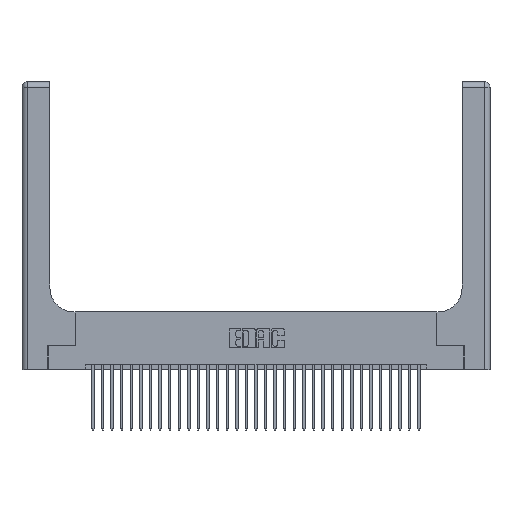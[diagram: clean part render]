
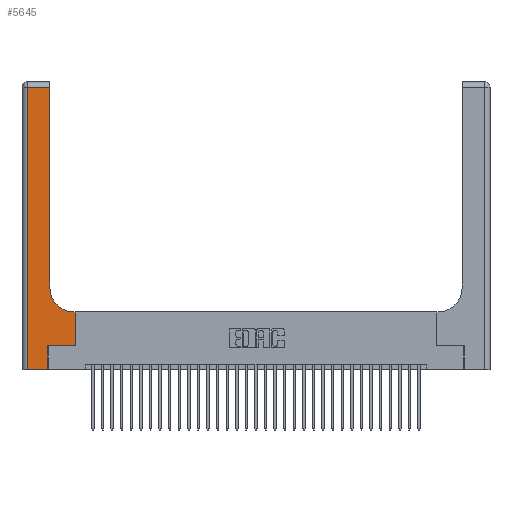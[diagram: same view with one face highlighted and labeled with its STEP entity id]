
A CAD part, top view. The second image highlights one B-rep face of the part: STEP entity #5645.
In plain terms, the highlighted planar face has unit normal (0, 0, 1).
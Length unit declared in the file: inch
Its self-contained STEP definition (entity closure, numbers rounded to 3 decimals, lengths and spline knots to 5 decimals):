
#362 = LINE ( 'NONE', #21223, #12542 ) ;
#438 = DIRECTION ( 'NONE',  ( -1., 0., 0. ) ) ;
#966 = LINE ( 'NONE', #25272, #27341 ) ;
#1006 = VECTOR ( 'NONE', #29697, 39.37008 ) ;
#2034 = CARTESIAN_POINT ( 'NONE',  ( 0., 3., 0.37 ) ) ;
#2257 = DIRECTION ( 'NONE',  ( 0., 0., -1. ) ) ;
#2410 = LINE ( 'NONE', #11811, #5665 ) ;
#4668 = LINE ( 'NONE', #6805, #24555 ) ;
#4976 = PLANE ( 'NONE',  #11623 ) ;
#5116 = AXIS2_PLACEMENT_3D ( 'NONE', #25966, #2257, #20649 ) ;
#5642 = CARTESIAN_POINT ( 'NONE',  ( 0.5585, 0.6, 0.37 ) ) ;
#5645 = ADVANCED_FACE ( 'NONE', ( #11794 ), #4976, .F. ) ;
#5660 = DIRECTION ( 'NONE',  ( 0., 1., 0. ) ) ;
#5665 = VECTOR ( 'NONE', #17160, 39.37008 ) ;
#6805 = CARTESIAN_POINT ( 'NONE',  ( 0.2915, 0.6, 0.37 ) ) ;
#6862 = ORIENTED_EDGE ( 'NONE', *, *, #28179, .T. ) ;
#6946 = CARTESIAN_POINT ( 'NONE',  ( 0.2915, 0.85, 0.37 ) ) ;
#7874 = VERTEX_POINT ( 'NONE', #30846 ) ;
#8010 = DIRECTION ( 'NONE',  ( 0., -1., 0. ) ) ;
#8282 = DIRECTION ( 'NONE',  ( -1., 0., 0. ) ) ;
#8579 = EDGE_CURVE ( 'NONE', #19270, #33022, #14827, .T. ) ;
#10180 = DIRECTION ( 'NONE',  ( 0., 0., -1. ) ) ;
#10274 = LINE ( 'NONE', #23566, #16364 ) ;
#10667 = CARTESIAN_POINT ( 'NONE',  ( 0.06, 2.94, 0.37 ) ) ;
#11623 = AXIS2_PLACEMENT_3D ( 'NONE', #2034, #10180, #438 ) ;
#11794 = FACE_OUTER_BOUND ( 'NONE', #29673, .T. ) ;
#11811 = CARTESIAN_POINT ( 'NONE',  ( 0.269, 0.25, 0.37 ) ) ;
#12025 = CARTESIAN_POINT ( 'NONE',  ( 0.269, 0., 0.37 ) ) ;
#12198 = ORIENTED_EDGE ( 'NONE', *, *, #13707, .T. ) ;
#12542 = VECTOR ( 'NONE', #8282, 39.37008 ) ;
#13707 = EDGE_CURVE ( 'NONE', #28319, #20152, #4668, .T. ) ;
#13866 = ORIENTED_EDGE ( 'NONE', *, *, #27782, .T. ) ;
#13912 = ORIENTED_EDGE ( 'NONE', *, *, #21150, .T. ) ;
#14245 = CARTESIAN_POINT ( 'NONE',  ( 0.06, 0., 0.37 ) ) ;
#14624 = DIRECTION ( 'NONE',  ( -1., 0., 0. ) ) ;
#14827 = LINE ( 'NONE', #31269, #1006 ) ;
#14865 = DIRECTION ( 'NONE',  ( 0., 1., 0. ) ) ;
#16364 = VECTOR ( 'NONE', #8010, 39.37008 ) ;
#16422 = LINE ( 'NONE', #12025, #25369 ) ;
#16515 = CIRCLE ( 'NONE', #5116, 0.25 ) ;
#16866 = ORIENTED_EDGE ( 'NONE', *, *, #21782, .T. ) ;
#17160 = DIRECTION ( 'NONE',  ( 1., 0., 0. ) ) ;
#17388 = EDGE_CURVE ( 'NONE', #28752, #7874, #2410, .T. ) ;
#17600 = VERTEX_POINT ( 'NONE', #29183 ) ;
#18431 = ORIENTED_EDGE ( 'NONE', *, *, #21505, .T. ) ;
#19270 = VERTEX_POINT ( 'NONE', #14245 ) ;
#20152 = VERTEX_POINT ( 'NONE', #30348 ) ;
#20291 = DIRECTION ( 'NONE',  ( 0., 1., 0. ) ) ;
#20379 = CARTESIAN_POINT ( 'NONE',  ( 0.269, 0.25, 0.37 ) ) ;
#20649 = DIRECTION ( 'NONE',  ( 1., 0., 0. ) ) ;
#21150 = EDGE_CURVE ( 'NONE', #7874, #28319, #29809, .T. ) ;
#21223 = CARTESIAN_POINT ( 'NONE',  ( 0., 2.94, 0.37 ) ) ;
#21505 = EDGE_CURVE ( 'NONE', #30972, #17600, #966, .T. ) ;
#21782 = EDGE_CURVE ( 'NONE', #30603, #19270, #10274, .T. ) ;
#23272 = ORIENTED_EDGE ( 'NONE', *, *, #8579, .T. ) ;
#23566 = CARTESIAN_POINT ( 'NONE',  ( 0.06, 3., 0.37 ) ) ;
#24555 = VECTOR ( 'NONE', #14624, 39.37008 ) ;
#25095 = ORIENTED_EDGE ( 'NONE', *, *, #29710, .T. ) ;
#25272 = CARTESIAN_POINT ( 'NONE',  ( 0.2915, 3., 0.37 ) ) ;
#25369 = VECTOR ( 'NONE', #14865, 39.37008 ) ;
#25966 = CARTESIAN_POINT ( 'NONE',  ( 0.5415, 0.85, 0.37 ) ) ;
#26417 = CARTESIAN_POINT ( 'NONE',  ( 0.5585, 0.25, 0.37 ) ) ;
#27341 = VECTOR ( 'NONE', #20291, 39.37008 ) ;
#27782 = EDGE_CURVE ( 'NONE', #17600, #30603, #362, .T. ) ;
#28179 = EDGE_CURVE ( 'NONE', #20152, #30972, #16515, .T. ) ;
#28319 = VERTEX_POINT ( 'NONE', #5642 ) ;
#28752 = VERTEX_POINT ( 'NONE', #20379 ) ;
#29183 = CARTESIAN_POINT ( 'NONE',  ( 0.2915, 2.94, 0.37 ) ) ;
#29226 = ORIENTED_EDGE ( 'NONE', *, *, #17388, .T. ) ;
#29673 = EDGE_LOOP ( 'NONE', ( #18431, #13866, #16866, #23272, #25095, #29226, #13912, #12198, #6862 ) ) ;
#29697 = DIRECTION ( 'NONE',  ( 1., 0., 0. ) ) ;
#29710 = EDGE_CURVE ( 'NONE', #33022, #28752, #16422, .T. ) ;
#29809 = LINE ( 'NONE', #26417, #31470 ) ;
#30348 = CARTESIAN_POINT ( 'NONE',  ( 0.5415, 0.6, 0.37 ) ) ;
#30603 = VERTEX_POINT ( 'NONE', #10667 ) ;
#30846 = CARTESIAN_POINT ( 'NONE',  ( 0.5585, 0.25, 0.37 ) ) ;
#30972 = VERTEX_POINT ( 'NONE', #6946 ) ;
#31269 = CARTESIAN_POINT ( 'NONE',  ( 0., 0., 0.37 ) ) ;
#31470 = VECTOR ( 'NONE', #5660, 39.37008 ) ;
#32936 = CARTESIAN_POINT ( 'NONE',  ( 0.269, 0., 0.37 ) ) ;
#33022 = VERTEX_POINT ( 'NONE', #32936 ) ;
